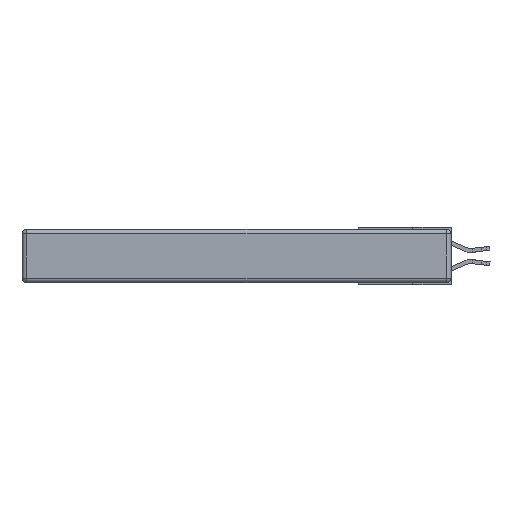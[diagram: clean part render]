
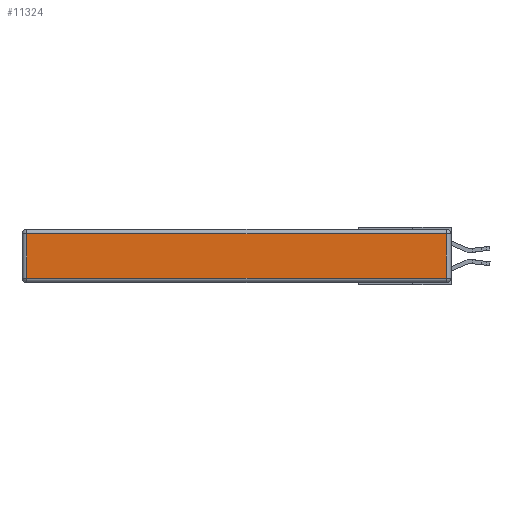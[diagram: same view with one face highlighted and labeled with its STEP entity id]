
A CAD part, left-side view. The second image highlights one B-rep face of the part: STEP entity #11324.
In plain terms, the highlighted planar face has unit normal (-1, 0, 0).
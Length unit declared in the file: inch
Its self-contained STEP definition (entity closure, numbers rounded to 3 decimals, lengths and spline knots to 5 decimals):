
#910 = CARTESIAN_POINT ( 'NONE',  ( 0., 2.72, -0.343 ) ) ;
#1255 = CARTESIAN_POINT ( 'NONE',  ( 0., 0.03, -0.03 ) ) ;
#1385 = VERTEX_POINT ( 'NONE', #1255 ) ;
#2513 = AXIS2_PLACEMENT_3D ( 'NONE', #15163, #7253, #8614 ) ;
#2892 = VERTEX_POINT ( 'NONE', #7755 ) ;
#3004 = CARTESIAN_POINT ( 'NONE',  ( 0., 2.72, -0.313 ) ) ;
#3897 = ORIENTED_EDGE ( 'NONE', *, *, #5917, .T. ) ;
#4298 = EDGE_CURVE ( 'NONE', #2892, #11685, #4800, .T. ) ;
#4800 = LINE ( 'NONE', #910, #11318 ) ;
#5255 = EDGE_LOOP ( 'NONE', ( #6018, #11683, #3897, #7848 ) ) ;
#5917 = EDGE_CURVE ( 'NONE', #1385, #2892, #7838, .T. ) ;
#6018 = ORIENTED_EDGE ( 'NONE', *, *, #12643, .T. ) ;
#7214 = CARTESIAN_POINT ( 'NONE',  ( 0., 0.03, -0.313 ) ) ;
#7253 = DIRECTION ( 'NONE',  ( -1., 0., 0. ) ) ;
#7415 = DIRECTION ( 'NONE',  ( 0., 0., -1. ) ) ;
#7599 = CARTESIAN_POINT ( 'NONE',  ( 0., 0., -0.313 ) ) ;
#7755 = CARTESIAN_POINT ( 'NONE',  ( 0., 2.72, -0.03 ) ) ;
#7838 = LINE ( 'NONE', #16796, #16362 ) ;
#7848 = ORIENTED_EDGE ( 'NONE', *, *, #4298, .T. ) ;
#8614 = DIRECTION ( 'NONE',  ( 0., 0., 1. ) ) ;
#9159 = FACE_OUTER_BOUND ( 'NONE', #5255, .T. ) ;
#11318 = VECTOR ( 'NONE', #7415, 39.37008 ) ;
#11324 = ADVANCED_FACE ( 'NONE', ( #9159 ), #12471, .T. ) ;
#11380 = DIRECTION ( 'NONE',  ( 0., 0., 1. ) ) ;
#11564 = LINE ( 'NONE', #11617, #13224 ) ;
#11572 = DIRECTION ( 'NONE',  ( 0., -1., 0. ) ) ;
#11603 = DIRECTION ( 'NONE',  ( 0., 1., 0. ) ) ;
#11617 = CARTESIAN_POINT ( 'NONE',  ( 0., 0.03, -0.343 ) ) ;
#11683 = ORIENTED_EDGE ( 'NONE', *, *, #12438, .T. ) ;
#11685 = VERTEX_POINT ( 'NONE', #3004 ) ;
#12152 = LINE ( 'NONE', #7599, #16236 ) ;
#12438 = EDGE_CURVE ( 'NONE', #16421, #1385, #11564, .T. ) ;
#12471 = PLANE ( 'NONE',  #2513 ) ;
#12643 = EDGE_CURVE ( 'NONE', #11685, #16421, #12152, .T. ) ;
#13224 = VECTOR ( 'NONE', #11380, 39.37008 ) ;
#15163 = CARTESIAN_POINT ( 'NONE',  ( 0., 0., -0.343 ) ) ;
#16236 = VECTOR ( 'NONE', #11572, 39.37008 ) ;
#16362 = VECTOR ( 'NONE', #11603, 39.37008 ) ;
#16421 = VERTEX_POINT ( 'NONE', #7214 ) ;
#16796 = CARTESIAN_POINT ( 'NONE',  ( 0., 2.75, -0.03 ) ) ;
